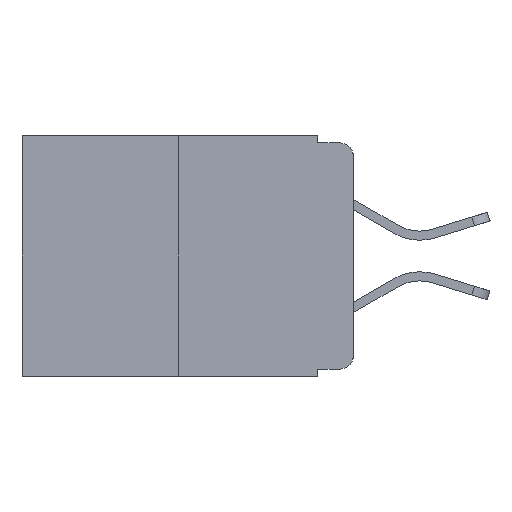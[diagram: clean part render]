
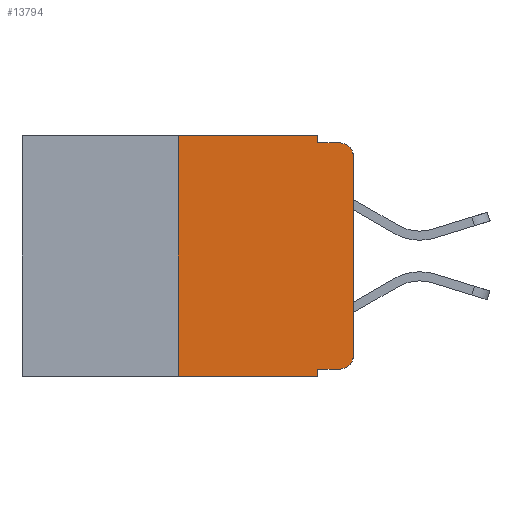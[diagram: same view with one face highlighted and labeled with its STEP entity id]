
A CAD part, left-side view. The second image highlights one B-rep face of the part: STEP entity #13794.
In plain terms, the highlighted planar face has unit normal (-1, 0, 0).
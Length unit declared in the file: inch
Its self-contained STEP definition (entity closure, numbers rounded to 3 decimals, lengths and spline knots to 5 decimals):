
#64 = CARTESIAN_POINT ( 'NONE',  ( 0., 0.25, -0.343 ) ) ;
#260 = EDGE_CURVE ( 'NONE', #3525, #12679, #13086, .T. ) ;
#401 = ORIENTED_EDGE ( 'NONE', *, *, #14576, .T. ) ;
#559 = EDGE_CURVE ( 'NONE', #16891, #3525, #7866, .T. ) ;
#756 = VERTEX_POINT ( 'NONE', #3929 ) ;
#873 = CARTESIAN_POINT ( 'NONE',  ( 0., 0., -0.03 ) ) ;
#1497 = EDGE_CURVE ( 'NONE', #4233, #9932, #5441, .T. ) ;
#1717 = CARTESIAN_POINT ( 'NONE',  ( 0., 0.473, 0. ) ) ;
#2073 = CARTESIAN_POINT ( 'NONE',  ( 0., 0.02, -0.333 ) ) ;
#2243 = CARTESIAN_POINT ( 'NONE',  ( 0., 0.473, 0. ) ) ;
#2309 = DIRECTION ( 'NONE',  ( 0., -1., 0. ) ) ;
#2557 = LINE ( 'NONE', #14649, #19515 ) ;
#2916 = CARTESIAN_POINT ( 'NONE',  ( 0., 0.051, -0.01 ) ) ;
#3035 = FACE_OUTER_BOUND ( 'NONE', #9422, .T. ) ;
#3469 = CARTESIAN_POINT ( 'NONE',  ( 0., 0.051, -0.01 ) ) ;
#3492 = PLANE ( 'NONE',  #15186 ) ;
#3525 = VERTEX_POINT ( 'NONE', #16299 ) ;
#3929 = CARTESIAN_POINT ( 'NONE',  ( 0., 0.02, -0.01 ) ) ;
#4168 = VECTOR ( 'NONE', #6591, 39.37008 ) ;
#4191 = EDGE_CURVE ( 'NONE', #18088, #12574, #7215, .T. ) ;
#4233 = VERTEX_POINT ( 'NONE', #18437 ) ;
#4631 = VECTOR ( 'NONE', #11906, 39.37008 ) ;
#4720 = EDGE_CURVE ( 'NONE', #9932, #7141, #14015, .T. ) ;
#4996 = DIRECTION ( 'NONE',  ( 0., 0., 1. ) ) ;
#5056 = AXIS2_PLACEMENT_3D ( 'NONE', #7332, #18661, #9049 ) ;
#5441 = LINE ( 'NONE', #19693, #17486 ) ;
#6352 = CARTESIAN_POINT ( 'NONE',  ( 0., 0.051, 0. ) ) ;
#6591 = DIRECTION ( 'NONE',  ( 0., 0., -1. ) ) ;
#6606 = VECTOR ( 'NONE', #8617, 39.37008 ) ;
#6732 = VERTEX_POINT ( 'NONE', #873 ) ;
#7125 = ORIENTED_EDGE ( 'NONE', *, *, #11284, .F. ) ;
#7141 = VERTEX_POINT ( 'NONE', #13822 ) ;
#7215 = LINE ( 'NONE', #19598, #15454 ) ;
#7332 = CARTESIAN_POINT ( 'NONE',  ( 0., 0.02, -0.03 ) ) ;
#7507 = DIRECTION ( 'NONE',  ( -1., 0., 0. ) ) ;
#7866 = LINE ( 'NONE', #2243, #12334 ) ;
#7948 = EDGE_CURVE ( 'NONE', #12679, #756, #11104, .T. ) ;
#8110 = DIRECTION ( 'NONE',  ( 0., 0., 1. ) ) ;
#8617 = DIRECTION ( 'NONE',  ( 0., -1., 0. ) ) ;
#8643 = DIRECTION ( 'NONE',  ( 0., 0., -1. ) ) ;
#9049 = DIRECTION ( 'NONE',  ( 0., 0., -1. ) ) ;
#9143 = CIRCLE ( 'NONE', #5056, 0.02 ) ;
#9261 = ORIENTED_EDGE ( 'NONE', *, *, #4191, .T. ) ;
#9422 = EDGE_LOOP ( 'NONE', ( #19414, #401, #15643, #20327, #17597, #9893, #9261, #7125, #12928, #11638 ) ) ;
#9893 = ORIENTED_EDGE ( 'NONE', *, *, #15587, .F. ) ;
#9932 = VERTEX_POINT ( 'NONE', #2073 ) ;
#10733 = AXIS2_PLACEMENT_3D ( 'NONE', #17254, #7507, #18830 ) ;
#11104 = LINE ( 'NONE', #3469, #6606 ) ;
#11284 = EDGE_CURVE ( 'NONE', #4233, #12574, #20886, .T. ) ;
#11638 = ORIENTED_EDGE ( 'NONE', *, *, #4720, .T. ) ;
#11906 = DIRECTION ( 'NONE',  ( 0., 0., -1. ) ) ;
#12334 = VECTOR ( 'NONE', #2309, 39.37008 ) ;
#12574 = VERTEX_POINT ( 'NONE', #15934 ) ;
#12679 = VERTEX_POINT ( 'NONE', #2916 ) ;
#12928 = ORIENTED_EDGE ( 'NONE', *, *, #1497, .T. ) ;
#13086 = LINE ( 'NONE', #6352, #4168 ) ;
#13794 = ADVANCED_FACE ( 'NONE', ( #3035 ), #3492, .F. ) ;
#13822 = CARTESIAN_POINT ( 'NONE',  ( 0., 0., -0.313 ) ) ;
#14015 = CIRCLE ( 'NONE', #10733, 0.02 ) ;
#14212 = VECTOR ( 'NONE', #4996, 39.37008 ) ;
#14576 = EDGE_CURVE ( 'NONE', #6732, #756, #9143, .T. ) ;
#14649 = CARTESIAN_POINT ( 'NONE',  ( 0., 0., 0. ) ) ;
#15186 = AXIS2_PLACEMENT_3D ( 'NONE', #1717, #18300, #8643 ) ;
#15454 = VECTOR ( 'NONE', #16246, 39.37008 ) ;
#15587 = EDGE_CURVE ( 'NONE', #18088, #16891, #18871, .T. ) ;
#15643 = ORIENTED_EDGE ( 'NONE', *, *, #7948, .F. ) ;
#15934 = CARTESIAN_POINT ( 'NONE',  ( 0., 0.051, -0.343 ) ) ;
#16246 = DIRECTION ( 'NONE',  ( 0., -1., 0. ) ) ;
#16299 = CARTESIAN_POINT ( 'NONE',  ( 0., 0.051, 0. ) ) ;
#16523 = CARTESIAN_POINT ( 'NONE',  ( 0., 0.25, 0. ) ) ;
#16891 = VERTEX_POINT ( 'NONE', #20024 ) ;
#17254 = CARTESIAN_POINT ( 'NONE',  ( 0., 0.02, -0.313 ) ) ;
#17486 = VECTOR ( 'NONE', #19719, 39.37008 ) ;
#17597 = ORIENTED_EDGE ( 'NONE', *, *, #559, .F. ) ;
#17850 = EDGE_CURVE ( 'NONE', #7141, #6732, #2557, .T. ) ;
#18088 = VERTEX_POINT ( 'NONE', #64 ) ;
#18300 = DIRECTION ( 'NONE',  ( 1., 0., 0. ) ) ;
#18437 = CARTESIAN_POINT ( 'NONE',  ( 0., 0.051, -0.333 ) ) ;
#18661 = DIRECTION ( 'NONE',  ( -1., 0., 0. ) ) ;
#18830 = DIRECTION ( 'NONE',  ( 0., 0., -1. ) ) ;
#18871 = LINE ( 'NONE', #16523, #14212 ) ;
#19414 = ORIENTED_EDGE ( 'NONE', *, *, #17850, .T. ) ;
#19515 = VECTOR ( 'NONE', #8110, 39.37008 ) ;
#19598 = CARTESIAN_POINT ( 'NONE',  ( 0., 0.473, -0.343 ) ) ;
#19693 = CARTESIAN_POINT ( 'NONE',  ( 0., 0.051, -0.333 ) ) ;
#19719 = DIRECTION ( 'NONE',  ( 0., -1., 0. ) ) ;
#20024 = CARTESIAN_POINT ( 'NONE',  ( 0., 0.25, 0. ) ) ;
#20327 = ORIENTED_EDGE ( 'NONE', *, *, #260, .F. ) ;
#20886 = LINE ( 'NONE', #21332, #4631 ) ;
#21332 = CARTESIAN_POINT ( 'NONE',  ( 0., 0.051, 0. ) ) ;
